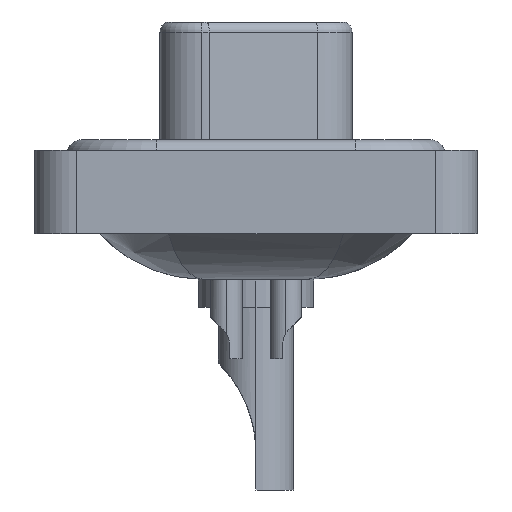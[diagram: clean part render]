
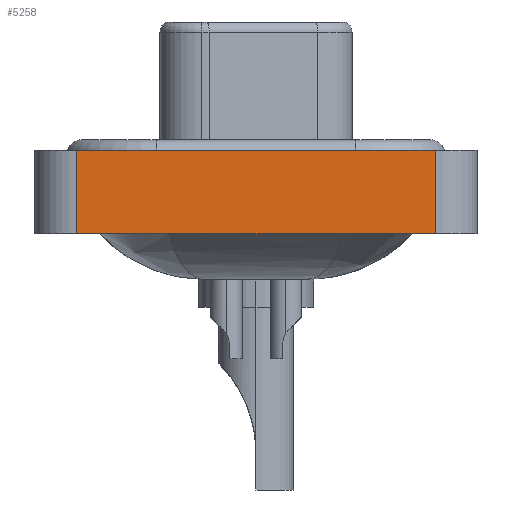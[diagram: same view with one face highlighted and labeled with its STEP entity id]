
A CAD part, left-side view. The second image highlights one B-rep face of the part: STEP entity #5258.
In plain terms, the highlighted planar face has unit normal (-1, 0, 0).
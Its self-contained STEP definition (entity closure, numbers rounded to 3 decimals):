
#110 = DIRECTION ( 'NONE',  ( 0., -1., 0. ) ) ;
#778 = DIRECTION ( 'NONE',  ( -1., 0., 0. ) ) ;
#1299 = EDGE_LOOP ( 'NONE', ( #19869, #10857, #12269, #11716 ) ) ;
#1386 = CARTESIAN_POINT ( 'NONE',  ( -7.3, -8.55, -3.6 ) ) ;
#3497 = FACE_OUTER_BOUND ( 'NONE', #1299, .T. ) ;
#3876 = LINE ( 'NONE', #18833, #15477 ) ;
#4711 = DIRECTION ( 'NONE',  ( 0., 0., 1. ) ) ;
#5258 = ADVANCED_FACE ( 'NONE', ( #3497 ), #8571, .T. ) ;
#5904 = VECTOR ( 'NONE', #110, 1000. ) ;
#5983 = CARTESIAN_POINT ( 'NONE',  ( -7.3, -8.55, -3.6 ) ) ;
#7617 = CARTESIAN_POINT ( 'NONE',  ( -7.3, 8.55, 0.4 ) ) ;
#8000 = LINE ( 'NONE', #21083, #5904 ) ;
#8090 = VECTOR ( 'NONE', #4711, 1000. ) ;
#8387 = LINE ( 'NONE', #1386, #8090 ) ;
#8571 = PLANE ( 'NONE',  #17937 ) ;
#8595 = DIRECTION ( 'NONE',  ( 0., -1., 0. ) ) ;
#10464 = DIRECTION ( 'NONE',  ( 0., 0., 1. ) ) ;
#10641 = EDGE_CURVE ( 'NONE', #19966, #12830, #3876, .T. ) ;
#10857 = ORIENTED_EDGE ( 'NONE', *, *, #19577, .F. ) ;
#11716 = ORIENTED_EDGE ( 'NONE', *, *, #21063, .T. ) ;
#12269 = ORIENTED_EDGE ( 'NONE', *, *, #10641, .F. ) ;
#12283 = CARTESIAN_POINT ( 'NONE',  ( -7.3, -8.55, 0.4 ) ) ;
#12830 = VERTEX_POINT ( 'NONE', #7617 ) ;
#13472 = VERTEX_POINT ( 'NONE', #15572 ) ;
#13758 = EDGE_CURVE ( 'NONE', #14554, #13472, #8387, .T. ) ;
#14554 = VERTEX_POINT ( 'NONE', #5983 ) ;
#15416 = CARTESIAN_POINT ( 'NONE',  ( -7.3, 8.55, -3.6 ) ) ;
#15447 = LINE ( 'NONE', #12283, #16850 ) ;
#15477 = VECTOR ( 'NONE', #10464, 1000. ) ;
#15572 = CARTESIAN_POINT ( 'NONE',  ( -7.3, -8.55, 0.4 ) ) ;
#16850 = VECTOR ( 'NONE', #8595, 1000. ) ;
#17245 = CARTESIAN_POINT ( 'NONE',  ( -7.3, -8.55, -3.6 ) ) ;
#17937 = AXIS2_PLACEMENT_3D ( 'NONE', #17245, #778, #18454 ) ;
#18454 = DIRECTION ( 'NONE',  ( 0., 0., 1. ) ) ;
#18833 = CARTESIAN_POINT ( 'NONE',  ( -7.3, 8.55, -3.6 ) ) ;
#19577 = EDGE_CURVE ( 'NONE', #12830, #13472, #15447, .T. ) ;
#19869 = ORIENTED_EDGE ( 'NONE', *, *, #13758, .T. ) ;
#19966 = VERTEX_POINT ( 'NONE', #15416 ) ;
#21063 = EDGE_CURVE ( 'NONE', #19966, #14554, #8000, .T. ) ;
#21083 = CARTESIAN_POINT ( 'NONE',  ( -7.3, -8.55, -3.6 ) ) ;
